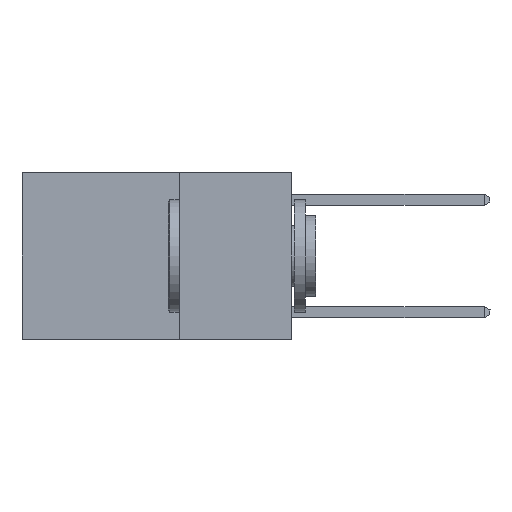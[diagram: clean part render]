
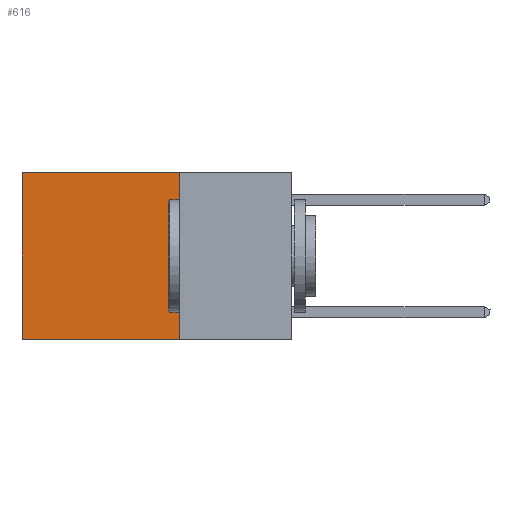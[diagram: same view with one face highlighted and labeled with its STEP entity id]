
A CAD part, left-side view. The second image highlights one B-rep face of the part: STEP entity #616.
In plain terms, the highlighted planar face has unit normal (-1, 0, 0).
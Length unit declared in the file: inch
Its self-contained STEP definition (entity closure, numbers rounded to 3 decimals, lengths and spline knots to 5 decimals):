
#80 = CARTESIAN_POINT ( 'NONE',  ( 0.2625, 0.6, -0.37 ) ) ;
#454 = CARTESIAN_POINT ( 'NONE',  ( 0.2625, 0.25, -0.37 ) ) ;
#616 = ADVANCED_FACE ( 'NONE', ( #7303 ), #12467, .F. ) ;
#667 = EDGE_CURVE ( 'NONE', #3294, #1383, #12360, .T. ) ;
#812 = EDGE_CURVE ( 'NONE', #3294, #13664, #3226, .T. ) ;
#1290 = ORIENTED_EDGE ( 'NONE', *, *, #13906, .T. ) ;
#1383 = VERTEX_POINT ( 'NONE', #12205 ) ;
#1481 = VERTEX_POINT ( 'NONE', #80 ) ;
#1572 = CARTESIAN_POINT ( 'NONE',  ( 0.2625, 0.25, 0. ) ) ;
#2588 = ORIENTED_EDGE ( 'NONE', *, *, #667, .F. ) ;
#3226 = LINE ( 'NONE', #11277, #8180 ) ;
#3294 = VERTEX_POINT ( 'NONE', #5856 ) ;
#4128 = LINE ( 'NONE', #454, #12820 ) ;
#4755 = CARTESIAN_POINT ( 'NONE',  ( 0.2625, 0.6, 0. ) ) ;
#4881 = DIRECTION ( 'NONE',  ( 0., 0., -1. ) ) ;
#4952 = DIRECTION ( 'NONE',  ( 1., 0., 0. ) ) ;
#5856 = CARTESIAN_POINT ( 'NONE',  ( 0.2625, 0.25, 0. ) ) ;
#6534 = EDGE_LOOP ( 'NONE', ( #1290, #8811, #2588, #6565 ) ) ;
#6565 = ORIENTED_EDGE ( 'NONE', *, *, #812, .T. ) ;
#6610 = VECTOR ( 'NONE', #4881, 39.37008 ) ;
#6701 = VECTOR ( 'NONE', #6982, 39.37008 ) ;
#6982 = DIRECTION ( 'NONE',  ( 0., 0., -1. ) ) ;
#7303 = FACE_OUTER_BOUND ( 'NONE', #6534, .T. ) ;
#7381 = EDGE_CURVE ( 'NONE', #1383, #1481, #4128, .T. ) ;
#8180 = VECTOR ( 'NONE', #12195, 39.37008 ) ;
#8811 = ORIENTED_EDGE ( 'NONE', *, *, #7381, .F. ) ;
#8908 = CARTESIAN_POINT ( 'NONE',  ( 0.2625, 0.6, 0. ) ) ;
#9597 = LINE ( 'NONE', #4755, #6701 ) ;
#9622 = DIRECTION ( 'NONE',  ( 0., 0., -1. ) ) ;
#10348 = DIRECTION ( 'NONE',  ( 0., 1., 0. ) ) ;
#10391 = CARTESIAN_POINT ( 'NONE',  ( 0.2625, 0.25, 0. ) ) ;
#11277 = CARTESIAN_POINT ( 'NONE',  ( 0.2625, 0.25, 0. ) ) ;
#12195 = DIRECTION ( 'NONE',  ( 0., 1., 0. ) ) ;
#12205 = CARTESIAN_POINT ( 'NONE',  ( 0.2625, 0.25, -0.37 ) ) ;
#12360 = LINE ( 'NONE', #1572, #6610 ) ;
#12407 = AXIS2_PLACEMENT_3D ( 'NONE', #10391, #4952, #9622 ) ;
#12467 = PLANE ( 'NONE',  #12407 ) ;
#12820 = VECTOR ( 'NONE', #10348, 39.37008 ) ;
#13664 = VERTEX_POINT ( 'NONE', #8908 ) ;
#13906 = EDGE_CURVE ( 'NONE', #13664, #1481, #9597, .T. ) ;
